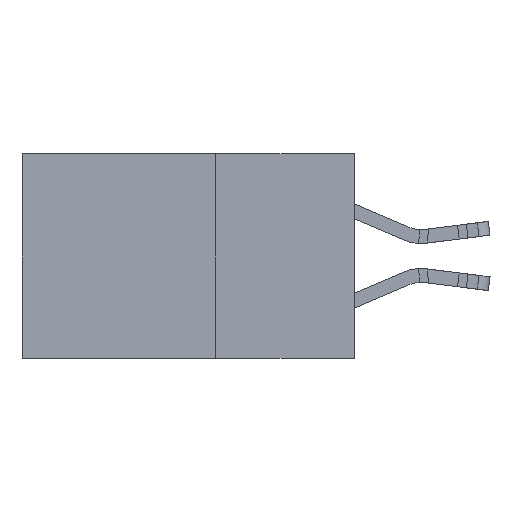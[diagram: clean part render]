
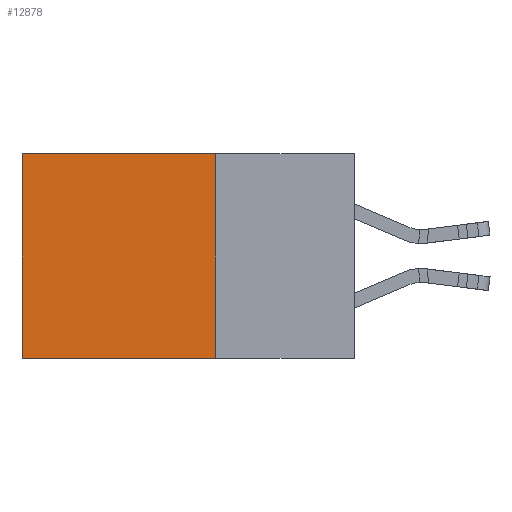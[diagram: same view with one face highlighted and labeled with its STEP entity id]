
A CAD part, left-side view. The second image highlights one B-rep face of the part: STEP entity #12878.
In plain terms, the highlighted planar face has unit normal (-1, 0, 0).
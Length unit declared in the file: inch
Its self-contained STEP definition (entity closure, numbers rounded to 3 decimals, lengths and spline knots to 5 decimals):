
#867 = DIRECTION ( 'NONE',  ( 0., 1., 0. ) ) ;
#1190 = LINE ( 'NONE', #10647, #20666 ) ;
#1444 = VECTOR ( 'NONE', #2386, 39.37008 ) ;
#1549 = LINE ( 'NONE', #3256, #20432 ) ;
#1813 = VECTOR ( 'NONE', #21639, 39.37008 ) ;
#2266 = ORIENTED_EDGE ( 'NONE', *, *, #18386, .F. ) ;
#2386 = DIRECTION ( 'NONE',  ( 0., 0., -1. ) ) ;
#2954 = DIRECTION ( 'NONE',  ( 0., 1., 0. ) ) ;
#3256 = CARTESIAN_POINT ( 'NONE',  ( 0.2615, 0.25, 0. ) ) ;
#4192 = EDGE_CURVE ( 'NONE', #16285, #21357, #1549, .T. ) ;
#4770 = CARTESIAN_POINT ( 'NONE',  ( 0.2615, 0.25, 0. ) ) ;
#4823 = CARTESIAN_POINT ( 'NONE',  ( 0.2615, 0.25, -0.37 ) ) ;
#6631 = CARTESIAN_POINT ( 'NONE',  ( 0.2615, 0.25, -0.37 ) ) ;
#6653 = EDGE_LOOP ( 'NONE', ( #11880, #2266, #13036, #20902 ) ) ;
#8557 = DIRECTION ( 'NONE',  ( 0., 0., -1. ) ) ;
#9653 = CARTESIAN_POINT ( 'NONE',  ( 0.2615, 0.6, -0.37 ) ) ;
#10296 = VERTEX_POINT ( 'NONE', #24242 ) ;
#10647 = CARTESIAN_POINT ( 'NONE',  ( 0.2615, 0.25, -0.37 ) ) ;
#11880 = ORIENTED_EDGE ( 'NONE', *, *, #12748, .T. ) ;
#11925 = AXIS2_PLACEMENT_3D ( 'NONE', #6631, #19683, #8557 ) ;
#12748 = EDGE_CURVE ( 'NONE', #21357, #16639, #20901, .T. ) ;
#12878 = ADVANCED_FACE ( 'NONE', ( #18639 ), #17844, .F. ) ;
#13036 = ORIENTED_EDGE ( 'NONE', *, *, #18379, .F. ) ;
#15152 = CARTESIAN_POINT ( 'NONE',  ( 0.2615, 0.6, 0. ) ) ;
#15724 = CARTESIAN_POINT ( 'NONE',  ( 0.2615, 0.6, -0.37 ) ) ;
#16285 = VERTEX_POINT ( 'NONE', #4770 ) ;
#16639 = VERTEX_POINT ( 'NONE', #9653 ) ;
#17844 = PLANE ( 'NONE',  #11925 ) ;
#18379 = EDGE_CURVE ( 'NONE', #16285, #10296, #21799, .T. ) ;
#18386 = EDGE_CURVE ( 'NONE', #10296, #16639, #1190, .T. ) ;
#18639 = FACE_OUTER_BOUND ( 'NONE', #6653, .T. ) ;
#19683 = DIRECTION ( 'NONE',  ( 1., 0., 0. ) ) ;
#20432 = VECTOR ( 'NONE', #867, 39.37008 ) ;
#20666 = VECTOR ( 'NONE', #2954, 39.37008 ) ;
#20901 = LINE ( 'NONE', #15724, #1444 ) ;
#20902 = ORIENTED_EDGE ( 'NONE', *, *, #4192, .T. ) ;
#21357 = VERTEX_POINT ( 'NONE', #15152 ) ;
#21639 = DIRECTION ( 'NONE',  ( 0., 0., -1. ) ) ;
#21799 = LINE ( 'NONE', #4823, #1813 ) ;
#24242 = CARTESIAN_POINT ( 'NONE',  ( 0.2615, 0.25, -0.37 ) ) ;
